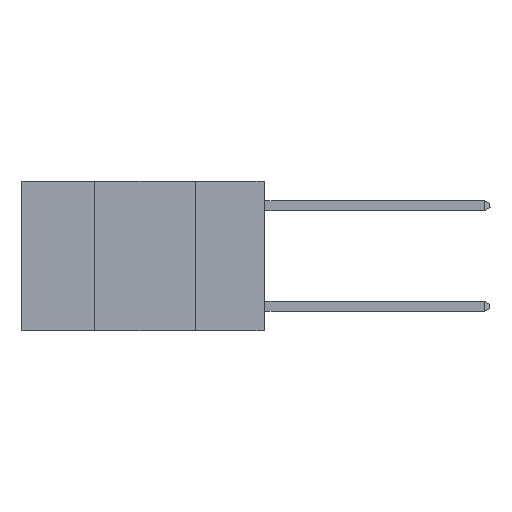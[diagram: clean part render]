
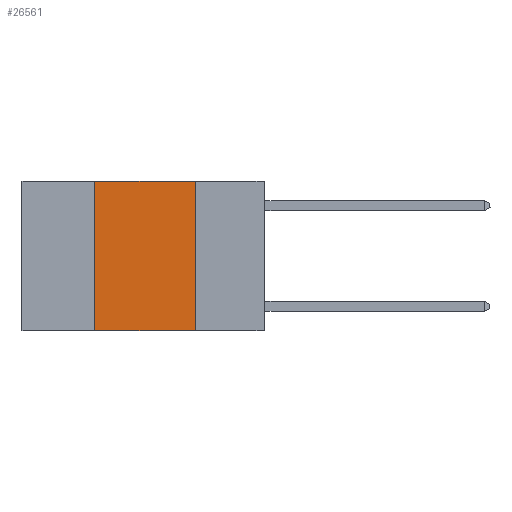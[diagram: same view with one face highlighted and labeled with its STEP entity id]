
A CAD part, left-side view. The second image highlights one B-rep face of the part: STEP entity #26561.
In plain terms, the highlighted planar face has unit normal (-1, 0, 0).
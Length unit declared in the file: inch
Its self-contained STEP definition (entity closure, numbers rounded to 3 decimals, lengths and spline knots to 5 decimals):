
#676 = DIRECTION ( 'NONE',  ( 1., 0., 0. ) ) ;
#1010 = CARTESIAN_POINT ( 'NONE',  ( 0., 0.6, -0.37 ) ) ;
#1072 = VECTOR ( 'NONE', #16771, 39.37008 ) ;
#1515 = VERTEX_POINT ( 'NONE', #19780 ) ;
#1851 = EDGE_LOOP ( 'NONE', ( #14881, #26698, #28338, #28374 ) ) ;
#2163 = FACE_OUTER_BOUND ( 'NONE', #1851, .T. ) ;
#3964 = CARTESIAN_POINT ( 'NONE',  ( 0., 0.17, 0. ) ) ;
#8240 = LINE ( 'NONE', #11864, #1072 ) ;
#8992 = EDGE_CURVE ( 'NONE', #17684, #1515, #8240, .T. ) ;
#11438 = LINE ( 'NONE', #21682, #30066 ) ;
#11864 = CARTESIAN_POINT ( 'NONE',  ( 0., 0.42, 0. ) ) ;
#12879 = EDGE_CURVE ( 'NONE', #17684, #25787, #28277, .T. ) ;
#14881 = ORIENTED_EDGE ( 'NONE', *, *, #16285, .F. ) ;
#16285 = EDGE_CURVE ( 'NONE', #28225, #25787, #24264, .T. ) ;
#16771 = DIRECTION ( 'NONE',  ( 0., 0., 1. ) ) ;
#17589 = DIRECTION ( 'NONE',  ( 0., 0., -1. ) ) ;
#17684 = VERTEX_POINT ( 'NONE', #30609 ) ;
#17737 = CARTESIAN_POINT ( 'NONE',  ( 0., 0.17, 0. ) ) ;
#19780 = CARTESIAN_POINT ( 'NONE',  ( 0., 0.42, 0. ) ) ;
#21682 = CARTESIAN_POINT ( 'NONE',  ( 0., 0.6, 0. ) ) ;
#21780 = VECTOR ( 'NONE', #27606, 39.37008 ) ;
#21802 = EDGE_CURVE ( 'NONE', #1515, #28225, #11438, .T. ) ;
#24110 = CARTESIAN_POINT ( 'NONE',  ( 0., 0.17, -0.37 ) ) ;
#24264 = LINE ( 'NONE', #3964, #29982 ) ;
#25005 = AXIS2_PLACEMENT_3D ( 'NONE', #29708, #676, #17589 ) ;
#25787 = VERTEX_POINT ( 'NONE', #24110 ) ;
#25813 = DIRECTION ( 'NONE',  ( 0., 0., -1. ) ) ;
#26561 = ADVANCED_FACE ( 'NONE', ( #2163 ), #27278, .F. ) ;
#26593 = DIRECTION ( 'NONE',  ( 0., -1., 0. ) ) ;
#26698 = ORIENTED_EDGE ( 'NONE', *, *, #21802, .F. ) ;
#27278 = PLANE ( 'NONE',  #25005 ) ;
#27606 = DIRECTION ( 'NONE',  ( 0., -1., 0. ) ) ;
#28225 = VERTEX_POINT ( 'NONE', #17737 ) ;
#28277 = LINE ( 'NONE', #1010, #21780 ) ;
#28338 = ORIENTED_EDGE ( 'NONE', *, *, #8992, .F. ) ;
#28374 = ORIENTED_EDGE ( 'NONE', *, *, #12879, .T. ) ;
#29708 = CARTESIAN_POINT ( 'NONE',  ( 0., 0.6, 0. ) ) ;
#29982 = VECTOR ( 'NONE', #25813, 39.37008 ) ;
#30066 = VECTOR ( 'NONE', #26593, 39.37008 ) ;
#30609 = CARTESIAN_POINT ( 'NONE',  ( 0., 0.42, -0.37 ) ) ;
